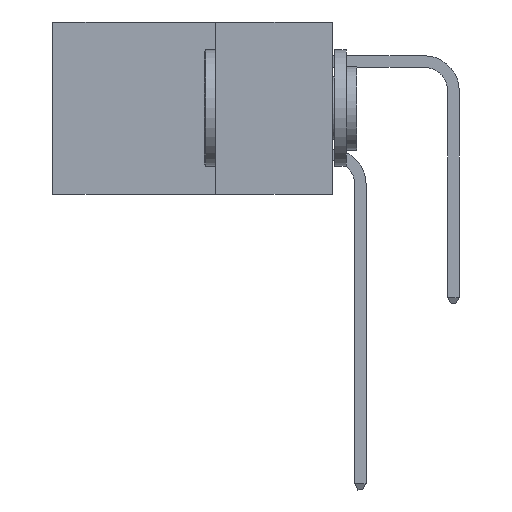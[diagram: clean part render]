
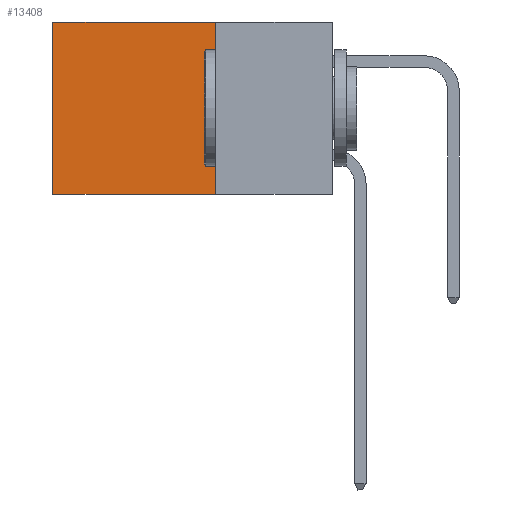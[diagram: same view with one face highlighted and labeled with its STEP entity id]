
A CAD part, left-side view. The second image highlights one B-rep face of the part: STEP entity #13408.
In plain terms, the highlighted planar face has unit normal (-1, 0, 0).
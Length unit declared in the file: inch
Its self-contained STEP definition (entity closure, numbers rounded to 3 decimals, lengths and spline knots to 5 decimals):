
#798 = CARTESIAN_POINT ( 'NONE',  ( 0.2615, 0.25, -0.37 ) ) ;
#1185 = ORIENTED_EDGE ( 'NONE', *, *, #14986, .F. ) ;
#1429 = VECTOR ( 'NONE', #21539, 39.37008 ) ;
#1597 = VERTEX_POINT ( 'NONE', #24706 ) ;
#2135 = CARTESIAN_POINT ( 'NONE',  ( 0.2615, 0.25, 0. ) ) ;
#2845 = LINE ( 'NONE', #19292, #1429 ) ;
#3079 = DIRECTION ( 'NONE',  ( 0., 0., -1. ) ) ;
#3820 = CARTESIAN_POINT ( 'NONE',  ( 0.2615, 0.6, 0. ) ) ;
#5820 = EDGE_LOOP ( 'NONE', ( #13693, #1185, #20173, #20924 ) ) ;
#6456 = VERTEX_POINT ( 'NONE', #2135 ) ;
#6824 = CARTESIAN_POINT ( 'NONE',  ( 0.2615, 0.6, -0.37 ) ) ;
#7378 = LINE ( 'NONE', #15110, #23813 ) ;
#7733 = VERTEX_POINT ( 'NONE', #12904 ) ;
#7917 = EDGE_CURVE ( 'NONE', #12977, #1597, #21128, .T. ) ;
#8343 = EDGE_CURVE ( 'NONE', #6456, #7733, #9901, .T. ) ;
#9901 = LINE ( 'NONE', #23921, #15836 ) ;
#10734 = DIRECTION ( 'NONE',  ( 0., 1., 0. ) ) ;
#12904 = CARTESIAN_POINT ( 'NONE',  ( 0.2615, 0.25, -0.37 ) ) ;
#12977 = VERTEX_POINT ( 'NONE', #3820 ) ;
#13408 = ADVANCED_FACE ( 'NONE', ( #17640 ), #14297, .F. ) ;
#13571 = EDGE_CURVE ( 'NONE', #6456, #12977, #2845, .T. ) ;
#13693 = ORIENTED_EDGE ( 'NONE', *, *, #7917, .T. ) ;
#14297 = PLANE ( 'NONE',  #16151 ) ;
#14986 = EDGE_CURVE ( 'NONE', #7733, #1597, #7378, .T. ) ;
#15110 = CARTESIAN_POINT ( 'NONE',  ( 0.2615, 0.25, -0.37 ) ) ;
#15836 = VECTOR ( 'NONE', #19549, 39.37008 ) ;
#16151 = AXIS2_PLACEMENT_3D ( 'NONE', #798, #16559, #3079 ) ;
#16559 = DIRECTION ( 'NONE',  ( 1., 0., 0. ) ) ;
#17640 = FACE_OUTER_BOUND ( 'NONE', #5820, .T. ) ;
#19292 = CARTESIAN_POINT ( 'NONE',  ( 0.2615, 0.25, 0. ) ) ;
#19549 = DIRECTION ( 'NONE',  ( 0., 0., -1. ) ) ;
#20160 = DIRECTION ( 'NONE',  ( 0., 0., -1. ) ) ;
#20173 = ORIENTED_EDGE ( 'NONE', *, *, #8343, .F. ) ;
#20420 = VECTOR ( 'NONE', #20160, 39.37008 ) ;
#20924 = ORIENTED_EDGE ( 'NONE', *, *, #13571, .T. ) ;
#21128 = LINE ( 'NONE', #6824, #20420 ) ;
#21539 = DIRECTION ( 'NONE',  ( 0., 1., 0. ) ) ;
#23813 = VECTOR ( 'NONE', #10734, 39.37008 ) ;
#23921 = CARTESIAN_POINT ( 'NONE',  ( 0.2615, 0.25, -0.37 ) ) ;
#24706 = CARTESIAN_POINT ( 'NONE',  ( 0.2615, 0.6, -0.37 ) ) ;
